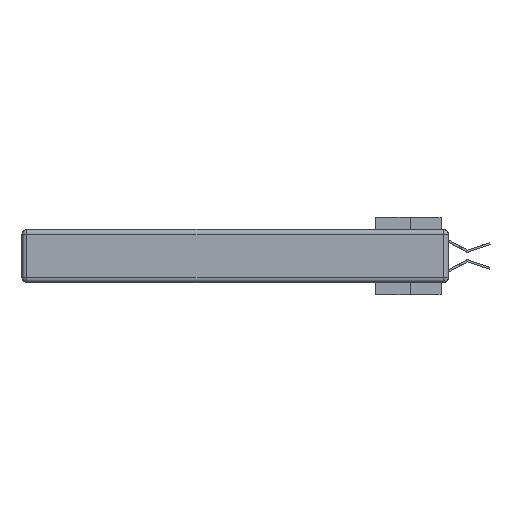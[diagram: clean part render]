
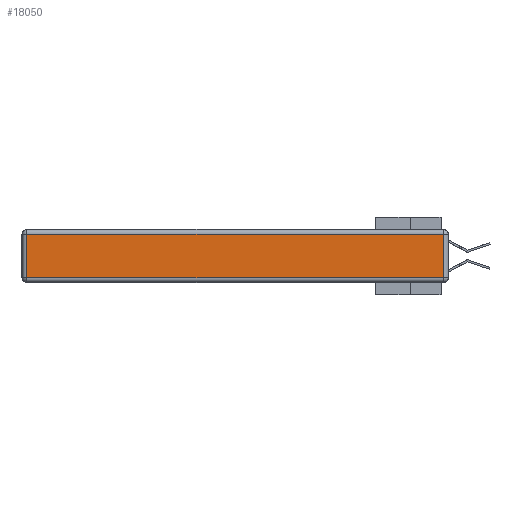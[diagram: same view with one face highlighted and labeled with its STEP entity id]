
A CAD part, left-side view. The second image highlights one B-rep face of the part: STEP entity #18050.
In plain terms, the highlighted planar face has unit normal (-1, 0, 0).
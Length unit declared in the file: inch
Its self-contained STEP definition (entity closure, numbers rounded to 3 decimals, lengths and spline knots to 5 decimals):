
#1269 = FACE_OUTER_BOUND ( 'NONE', #10322, .T. ) ;
#1802 = LINE ( 'NONE', #2332, #7449 ) ;
#1955 = EDGE_CURVE ( 'NONE', #5924, #3564, #23728, .T. ) ;
#2310 = DIRECTION ( 'NONE',  ( 0., 0., -1. ) ) ;
#2332 = CARTESIAN_POINT ( 'NONE',  ( 0., 2.75, -0.03 ) ) ;
#2999 = CARTESIAN_POINT ( 'NONE',  ( 0., 0., -0.343 ) ) ;
#3564 = VERTEX_POINT ( 'NONE', #16373 ) ;
#4257 = DIRECTION ( 'NONE',  ( 0., -1., 0. ) ) ;
#4856 = CARTESIAN_POINT ( 'NONE',  ( 0., 2.72, -0.343 ) ) ;
#5924 = VERTEX_POINT ( 'NONE', #30488 ) ;
#6110 = DIRECTION ( 'NONE',  ( 0., 0., 1. ) ) ;
#6759 = VECTOR ( 'NONE', #4257, 39.37008 ) ;
#7449 = VECTOR ( 'NONE', #16432, 39.37008 ) ;
#8955 = DIRECTION ( 'NONE',  ( -1., 0., 0. ) ) ;
#10322 = EDGE_LOOP ( 'NONE', ( #19376, #15927, #30103, #10679 ) ) ;
#10679 = ORIENTED_EDGE ( 'NONE', *, *, #1955, .T. ) ;
#13044 = EDGE_CURVE ( 'NONE', #3564, #16394, #20221, .T. ) ;
#14190 = DIRECTION ( 'NONE',  ( 0., 0., 1. ) ) ;
#15677 = EDGE_CURVE ( 'NONE', #16394, #20671, #33180, .T. ) ;
#15927 = ORIENTED_EDGE ( 'NONE', *, *, #15677, .T. ) ;
#16373 = CARTESIAN_POINT ( 'NONE',  ( 0., 2.72, -0.313 ) ) ;
#16394 = VERTEX_POINT ( 'NONE', #25668 ) ;
#16432 = DIRECTION ( 'NONE',  ( 0., 1., 0. ) ) ;
#18050 = ADVANCED_FACE ( 'NONE', ( #1269 ), #22699, .T. ) ;
#19376 = ORIENTED_EDGE ( 'NONE', *, *, #13044, .T. ) ;
#19602 = CARTESIAN_POINT ( 'NONE',  ( 0., 0.03, -0.343 ) ) ;
#20221 = LINE ( 'NONE', #21052, #6759 ) ;
#20671 = VERTEX_POINT ( 'NONE', #33431 ) ;
#21052 = CARTESIAN_POINT ( 'NONE',  ( 0., 0., -0.313 ) ) ;
#22699 = PLANE ( 'NONE',  #29184 ) ;
#23728 = LINE ( 'NONE', #4856, #34180 ) ;
#25668 = CARTESIAN_POINT ( 'NONE',  ( 0., 0.03, -0.313 ) ) ;
#25778 = VECTOR ( 'NONE', #6110, 39.37008 ) ;
#26919 = EDGE_CURVE ( 'NONE', #20671, #5924, #1802, .T. ) ;
#29184 = AXIS2_PLACEMENT_3D ( 'NONE', #2999, #8955, #14190 ) ;
#30103 = ORIENTED_EDGE ( 'NONE', *, *, #26919, .T. ) ;
#30488 = CARTESIAN_POINT ( 'NONE',  ( 0., 2.72, -0.03 ) ) ;
#33180 = LINE ( 'NONE', #19602, #25778 ) ;
#33431 = CARTESIAN_POINT ( 'NONE',  ( 0., 0.03, -0.03 ) ) ;
#34180 = VECTOR ( 'NONE', #2310, 39.37008 ) ;
